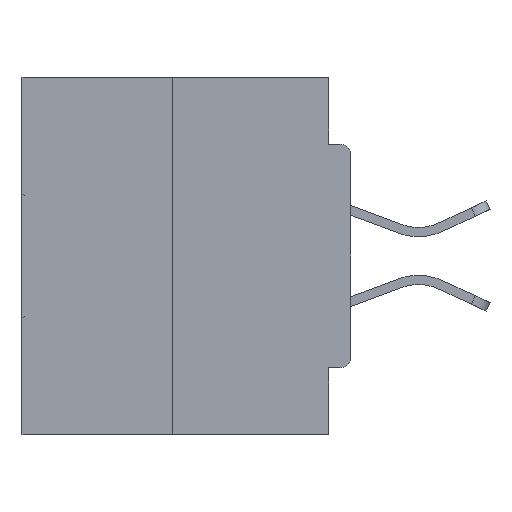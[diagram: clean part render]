
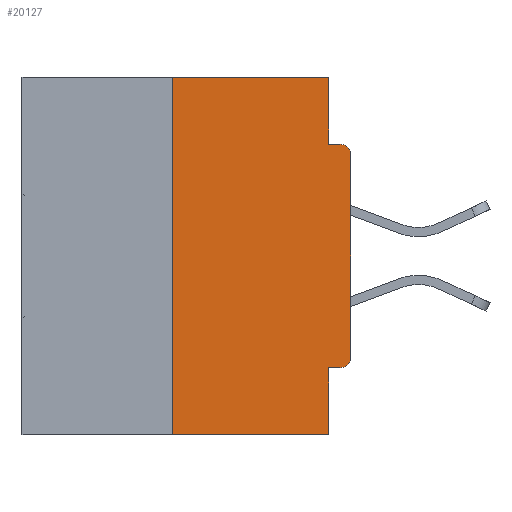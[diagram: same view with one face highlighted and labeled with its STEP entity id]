
A CAD part, left-side view. The second image highlights one B-rep face of the part: STEP entity #20127.
In plain terms, the highlighted planar face has unit normal (-1, 0, 0).
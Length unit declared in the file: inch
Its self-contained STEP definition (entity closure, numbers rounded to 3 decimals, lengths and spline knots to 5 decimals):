
#136 = CARTESIAN_POINT ( 'NONE',  ( 0., 0., -0.0935 ) ) ;
#364 = DIRECTION ( 'NONE',  ( 0., 0., -1. ) ) ;
#1555 = CARTESIAN_POINT ( 'NONE',  ( 0., 0.46, 0. ) ) ;
#1888 = LINE ( 'NONE', #23354, #9467 ) ;
#2072 = CARTESIAN_POINT ( 'NONE',  ( 0., 0., 0. ) ) ;
#2256 = VECTOR ( 'NONE', #24882, 39.37008 ) ;
#2269 = CARTESIAN_POINT ( 'NONE',  ( 0., 0., -0.4065 ) ) ;
#2516 = CARTESIAN_POINT ( 'NONE',  ( 0., 0.25, 0. ) ) ;
#6496 = ORIENTED_EDGE ( 'NONE', *, *, #28942, .F. ) ;
#6632 = DIRECTION ( 'NONE',  ( 0., 0., -1. ) ) ;
#7221 = DIRECTION ( 'NONE',  ( 0., -1., 0. ) ) ;
#7710 = ORIENTED_EDGE ( 'NONE', *, *, #15702, .T. ) ;
#8930 = LINE ( 'NONE', #2516, #29230 ) ;
#9467 = VECTOR ( 'NONE', #7221, 39.37008 ) ;
#10148 = DIRECTION ( 'NONE',  ( 0., 0., -1. ) ) ;
#10379 = VECTOR ( 'NONE', #10148, 39.37008 ) ;
#10724 = DIRECTION ( 'NONE',  ( 0., 0., -1. ) ) ;
#11391 = LINE ( 'NONE', #2072, #2256 ) ;
#11572 = EDGE_CURVE ( 'NONE', #24638, #24390, #34273, .T. ) ;
#11887 = DIRECTION ( 'NONE',  ( 0., 1., 0. ) ) ;
#13188 = VECTOR ( 'NONE', #27373, 39.37008 ) ;
#14196 = EDGE_CURVE ( 'NONE', #24390, #36065, #29855, .T. ) ;
#15266 = VECTOR ( 'NONE', #11887, 39.37008 ) ;
#15523 = CARTESIAN_POINT ( 'NONE',  ( 0., 0.015, -0.4065 ) ) ;
#15702 = EDGE_CURVE ( 'NONE', #20485, #36012, #26649, .T. ) ;
#16066 = AXIS2_PLACEMENT_3D ( 'NONE', #20505, #33025, #10724 ) ;
#16630 = ORIENTED_EDGE ( 'NONE', *, *, #14196, .F. ) ;
#16906 = VERTEX_POINT ( 'NONE', #33680 ) ;
#17510 = EDGE_CURVE ( 'NONE', #17785, #24638, #31587, .T. ) ;
#17785 = VERTEX_POINT ( 'NONE', #37968 ) ;
#18736 = FACE_OUTER_BOUND ( 'NONE', #19528, .T. ) ;
#19501 = CARTESIAN_POINT ( 'NONE',  ( 0., 0.015, -0.3915 ) ) ;
#19528 = EDGE_LOOP ( 'NONE', ( #37054, #6496, #20519, #38519, #19652, #7710, #31042, #38887, #16630, #22654 ) ) ;
#19652 = ORIENTED_EDGE ( 'NONE', *, *, #25316, .F. ) ;
#19782 = CARTESIAN_POINT ( 'NONE',  ( 0., 0.031, 0. ) ) ;
#19784 = DIRECTION ( 'NONE',  ( -1., 0., 0. ) ) ;
#19934 = PLANE ( 'NONE',  #16066 ) ;
#20127 = ADVANCED_FACE ( 'NONE', ( #18736 ), #19934, .F. ) ;
#20485 = VERTEX_POINT ( 'NONE', #15523 ) ;
#20505 = CARTESIAN_POINT ( 'NONE',  ( 0., 0.46, 0. ) ) ;
#20519 = ORIENTED_EDGE ( 'NONE', *, *, #41891, .T. ) ;
#20829 = CARTESIAN_POINT ( 'NONE',  ( 0., 0.031, -0.5 ) ) ;
#21605 = AXIS2_PLACEMENT_3D ( 'NONE', #39249, #19784, #364 ) ;
#22654 = ORIENTED_EDGE ( 'NONE', *, *, #11572, .F. ) ;
#23044 = DIRECTION ( 'NONE',  ( -1., 0., 0. ) ) ;
#23227 = EDGE_CURVE ( 'NONE', #36012, #16906, #11391, .T. ) ;
#23332 = LINE ( 'NONE', #2269, #15266 ) ;
#23354 = CARTESIAN_POINT ( 'NONE',  ( 0., 0.46, -0.5 ) ) ;
#23875 = VERTEX_POINT ( 'NONE', #36531 ) ;
#23936 = EDGE_CURVE ( 'NONE', #16906, #36065, #34681, .T. ) ;
#24390 = VERTEX_POINT ( 'NONE', #39334 ) ;
#24638 = VERTEX_POINT ( 'NONE', #34350 ) ;
#24731 = VERTEX_POINT ( 'NONE', #34900 ) ;
#24882 = DIRECTION ( 'NONE',  ( 0., 0., 1. ) ) ;
#24954 = CARTESIAN_POINT ( 'NONE',  ( 0., 0.015, -0.0935 ) ) ;
#25316 = EDGE_CURVE ( 'NONE', #20485, #35603, #23332, .T. ) ;
#26649 = CIRCLE ( 'NONE', #38276, 0.015 ) ;
#27373 = DIRECTION ( 'NONE',  ( 0., 0., -1. ) ) ;
#28942 = EDGE_CURVE ( 'NONE', #24731, #17785, #8930, .T. ) ;
#29230 = VECTOR ( 'NONE', #41273, 39.37008 ) ;
#29466 = LINE ( 'NONE', #20829, #13188 ) ;
#29855 = LINE ( 'NONE', #136, #37926 ) ;
#31042 = ORIENTED_EDGE ( 'NONE', *, *, #23227, .T. ) ;
#31163 = CARTESIAN_POINT ( 'NONE',  ( 0., 0.031, -0.4065 ) ) ;
#31587 = LINE ( 'NONE', #1555, #41251 ) ;
#32071 = EDGE_CURVE ( 'NONE', #35603, #23875, #29466, .T. ) ;
#33025 = DIRECTION ( 'NONE',  ( 1., 0., 0. ) ) ;
#33072 = DIRECTION ( 'NONE',  ( 0., -1., 0. ) ) ;
#33487 = DIRECTION ( 'NONE',  ( 0., -1., 0. ) ) ;
#33680 = CARTESIAN_POINT ( 'NONE',  ( 0., 0., -0.1085 ) ) ;
#34273 = LINE ( 'NONE', #19782, #10379 ) ;
#34350 = CARTESIAN_POINT ( 'NONE',  ( 0., 0.031, 0. ) ) ;
#34681 = CIRCLE ( 'NONE', #21605, 0.015 ) ;
#34900 = CARTESIAN_POINT ( 'NONE',  ( 0., 0.25, -0.5 ) ) ;
#35603 = VERTEX_POINT ( 'NONE', #31163 ) ;
#36012 = VERTEX_POINT ( 'NONE', #41300 ) ;
#36065 = VERTEX_POINT ( 'NONE', #24954 ) ;
#36531 = CARTESIAN_POINT ( 'NONE',  ( 0., 0.031, -0.5 ) ) ;
#37054 = ORIENTED_EDGE ( 'NONE', *, *, #17510, .F. ) ;
#37926 = VECTOR ( 'NONE', #33072, 39.37008 ) ;
#37968 = CARTESIAN_POINT ( 'NONE',  ( 0., 0.25, 0. ) ) ;
#38276 = AXIS2_PLACEMENT_3D ( 'NONE', #19501, #23044, #6632 ) ;
#38519 = ORIENTED_EDGE ( 'NONE', *, *, #32071, .F. ) ;
#38887 = ORIENTED_EDGE ( 'NONE', *, *, #23936, .T. ) ;
#39249 = CARTESIAN_POINT ( 'NONE',  ( 0., 0.015, -0.1085 ) ) ;
#39334 = CARTESIAN_POINT ( 'NONE',  ( 0., 0.031, -0.0935 ) ) ;
#41251 = VECTOR ( 'NONE', #33487, 39.37008 ) ;
#41273 = DIRECTION ( 'NONE',  ( 0., 0., 1. ) ) ;
#41300 = CARTESIAN_POINT ( 'NONE',  ( 0., 0., -0.3915 ) ) ;
#41891 = EDGE_CURVE ( 'NONE', #24731, #23875, #1888, .T. ) ;
